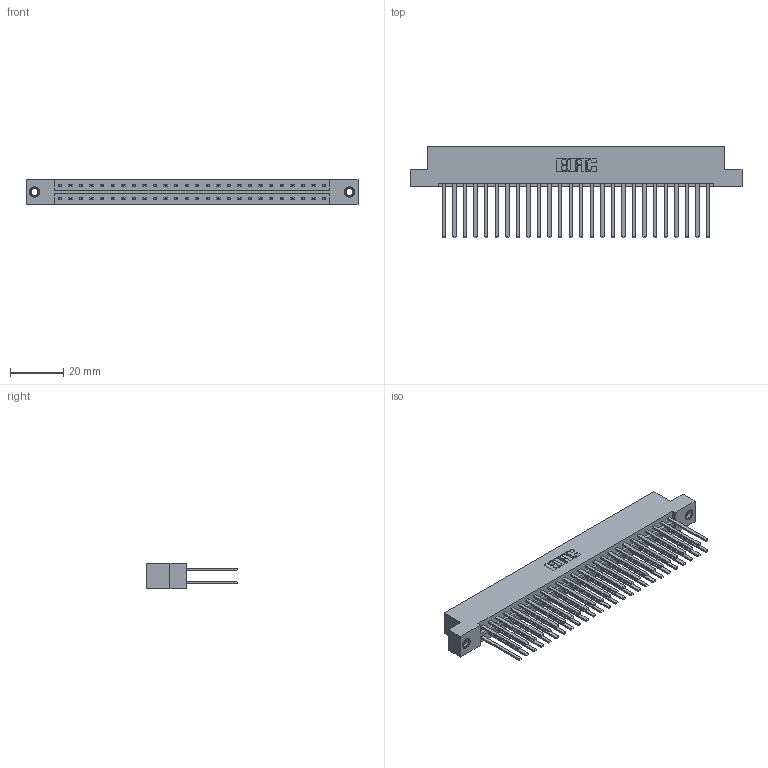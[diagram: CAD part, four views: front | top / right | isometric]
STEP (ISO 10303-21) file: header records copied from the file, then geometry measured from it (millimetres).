
FILE_DESCRIPTION (( 'STEP AP203' ), '1' );
FILE_NAME ('333-052-544-207.STEP', '2018-08-04T02:33:41', ( '' ), ( '' ), 'SwSTEP 2.0', 'SolidWorks 2016', '' );
FILE_SCHEMA (( 'CONFIG_CONTROL_DESIGN' ));
Length unit declared in the file: inch
Products named in the file (4): 333 Part_Flush - .156 Dia - TI; 345-292-001_345-293-144; 345-250-001_345-250-005-103; 333-052-544-207
Assembly tree (55 placements, depth 2):
  333-052-544-207
    333 Part_Flush - .156 Dia - TI
    345-292-001_345-293-144  x52
    345-250-001_345-250-005-103  x2
Bounding box: 124.56 x 34.3 x 9.4 mm (x, y, z)
Volume: 13282.8 mm3; surface area: 17912.8 mm2
Topology: 55 solids, 55 shells, 2566 faces, 7571 edges, 4970 vertices
Faces by surface type: plane 1766, cylinder 784, cone 12, torus 4
Entity records: 19798 total; most frequent: CARTESIAN_POINT 3281, ORIENTED_EDGE 3210, DIRECTION 2859, EDGE_CURVE 1605, VECTOR 1461, LINE 1461, VERTEX_POINT 1064, AXIS2_PLACEMENT_3D 699
